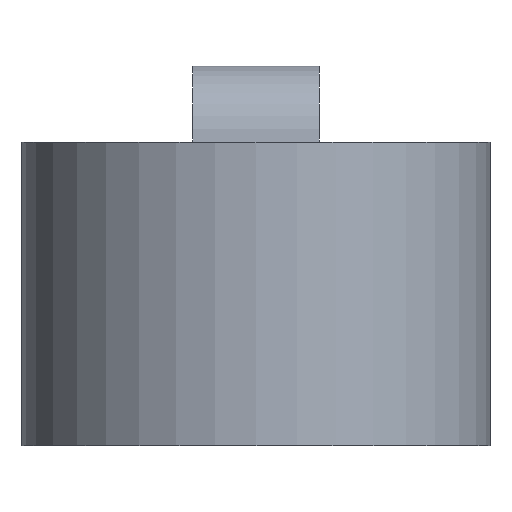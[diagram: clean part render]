
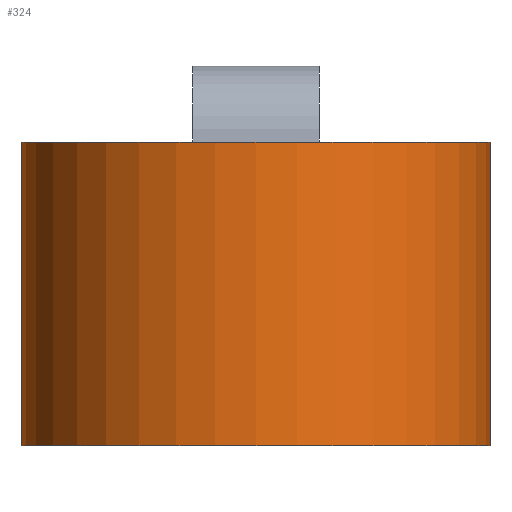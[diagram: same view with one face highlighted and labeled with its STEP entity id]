
A CAD part, front view. The second image highlights one B-rep face of the part: STEP entity #324.
In plain terms, the highlighted cylindrical face has radius 7.823 mm (diameter 15.646 mm), a partial arc.
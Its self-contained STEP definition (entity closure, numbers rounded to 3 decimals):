
#7 = ORIENTED_EDGE ( 'NONE', *, *, #227, .T. ) ;
#11 = EDGE_CURVE ( 'NONE', #62, #63, #98, .T. ) ;
#23 = EDGE_CURVE ( 'NONE', #276, #214, #56, .T. ) ;
#35 = EDGE_LOOP ( 'NONE', ( #249, #7, #71, #78 ) ) ;
#56 = LINE ( 'NONE', #262, #155 ) ;
#62 = VERTEX_POINT ( 'NONE', #310 ) ;
#63 = VERTEX_POINT ( 'NONE', #319 ) ;
#71 = ORIENTED_EDGE ( 'NONE', *, *, #11, .T. ) ;
#77 = CIRCLE ( 'NONE', #384, 7.823 ) ;
#78 = ORIENTED_EDGE ( 'NONE', *, *, #230, .T. ) ;
#98 = LINE ( 'NONE', #257, #166 ) ;
#99 = CARTESIAN_POINT ( 'NONE',  ( 0., 0., 2.54 ) ) ;
#102 = DIRECTION ( 'NONE',  ( -1., 0., 0. ) ) ;
#121 = CARTESIAN_POINT ( 'NONE',  ( 7.823, 0., 2.54 ) ) ;
#125 = DIRECTION ( 'NONE',  ( 0., 0., -1. ) ) ;
#126 = DIRECTION ( 'NONE',  ( 0., 0., 1. ) ) ;
#131 = DIRECTION ( 'NONE',  ( -1., 0., 0. ) ) ;
#140 = DIRECTION ( 'NONE',  ( 0., 0., -1. ) ) ;
#141 = CARTESIAN_POINT ( 'NONE',  ( 0., 0., -7.62 ) ) ;
#152 = DIRECTION ( 'NONE',  ( -1., 0., 0. ) ) ;
#153 = CARTESIAN_POINT ( 'NONE',  ( 0., 0., 2.54 ) ) ;
#155 = VECTOR ( 'NONE', #265, 1000. ) ;
#166 = VECTOR ( 'NONE', #253, 1000. ) ;
#167 = CARTESIAN_POINT ( 'NONE',  ( 7.823, 0., -7.62 ) ) ;
#214 = VERTEX_POINT ( 'NONE', #167 ) ;
#227 = EDGE_CURVE ( 'NONE', #276, #62, #420, .T. ) ;
#230 = EDGE_CURVE ( 'NONE', #63, #214, #77, .T. ) ;
#249 = ORIENTED_EDGE ( 'NONE', *, *, #23, .F. ) ;
#253 = DIRECTION ( 'NONE',  ( 0., 0., -1. ) ) ;
#257 = CARTESIAN_POINT ( 'NONE',  ( -7.823, 0., 2.54 ) ) ;
#262 = CARTESIAN_POINT ( 'NONE',  ( 7.823, 0., 2.54 ) ) ;
#265 = DIRECTION ( 'NONE',  ( 0., 0., -1. ) ) ;
#273 = CYLINDRICAL_SURFACE ( 'NONE', #360, 7.823 ) ;
#276 = VERTEX_POINT ( 'NONE', #121 ) ;
#310 = CARTESIAN_POINT ( 'NONE',  ( -7.823, 0., 2.54 ) ) ;
#319 = CARTESIAN_POINT ( 'NONE',  ( -7.823, 0., -7.62 ) ) ;
#324 = ADVANCED_FACE ( 'NONE', ( #428 ), #273, .T. ) ;
#360 = AXIS2_PLACEMENT_3D ( 'NONE', #99, #125, #102 ) ;
#384 = AXIS2_PLACEMENT_3D ( 'NONE', #141, #126, #131 ) ;
#405 = AXIS2_PLACEMENT_3D ( 'NONE', #153, #140, #152 ) ;
#420 = CIRCLE ( 'NONE', #405, 7.823 ) ;
#428 = FACE_OUTER_BOUND ( 'NONE', #35, .T. ) ;
